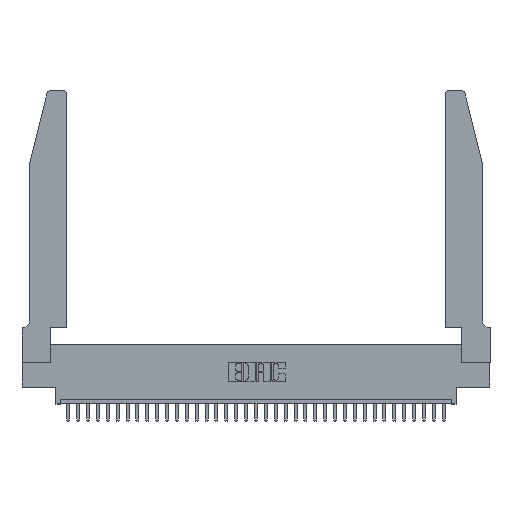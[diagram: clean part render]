
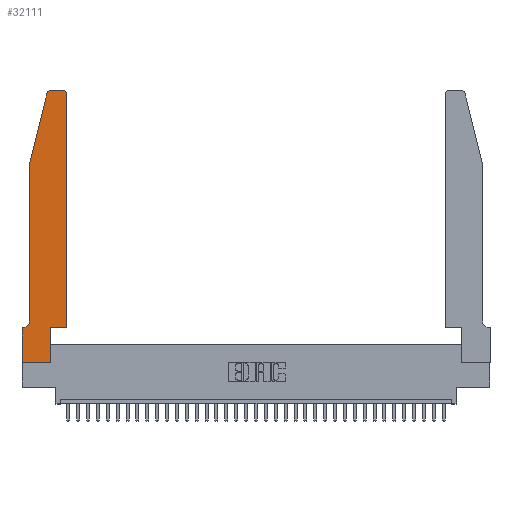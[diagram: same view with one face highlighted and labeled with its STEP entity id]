
A CAD part, top view. The second image highlights one B-rep face of the part: STEP entity #32111.
In plain terms, the highlighted planar face has unit normal (0, 0, 1).
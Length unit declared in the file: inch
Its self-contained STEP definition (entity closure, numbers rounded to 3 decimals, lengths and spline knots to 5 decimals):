
#231 = LINE ( 'NONE', #25158, #9953 ) ;
#695 = EDGE_CURVE ( 'NONE', #13591, #30207, #231, .T. ) ;
#723 = VERTEX_POINT ( 'NONE', #19340 ) ;
#740 = VERTEX_POINT ( 'NONE', #11806 ) ;
#1119 = EDGE_CURVE ( 'NONE', #15987, #22482, #8216, .T. ) ;
#1306 = VECTOR ( 'NONE', #20928, 39.37008 ) ;
#1535 = CARTESIAN_POINT ( 'NONE',  ( 0.0755, 2., 0.37 ) ) ;
#1785 = CARTESIAN_POINT ( 'NONE',  ( 0.4205, 2.72, 0.37 ) ) ;
#2062 = CARTESIAN_POINT ( 'NONE',  ( 0.2865, 0.35, 0.37 ) ) ;
#2480 = ORIENTED_EDGE ( 'NONE', *, *, #1119, .T. ) ;
#2664 = DIRECTION ( 'NONE',  ( 1., 0., 0. ) ) ;
#2764 = DIRECTION ( 'NONE',  ( 0., 0., 1. ) ) ;
#2852 = VERTEX_POINT ( 'NONE', #3169 ) ;
#2932 = EDGE_CURVE ( 'NONE', #723, #13591, #22415, .T. ) ;
#3169 = CARTESIAN_POINT ( 'NONE',  ( 0.0055, 0.35, 0.37 ) ) ;
#3414 = ORIENTED_EDGE ( 'NONE', *, *, #4445, .T. ) ;
#3510 = CARTESIAN_POINT ( 'NONE',  ( 0.25487, 2.72718, 0.37 ) ) ;
#3729 = AXIS2_PLACEMENT_3D ( 'NONE', #18151, #2764, #2664 ) ;
#4177 = EDGE_CURVE ( 'NONE', #9342, #21267, #10605, .T. ) ;
#4374 = DIRECTION ( 'NONE',  ( 0., -1., 0. ) ) ;
#4445 = EDGE_CURVE ( 'NONE', #21267, #28491, #19620, .T. ) ;
#4500 = DIRECTION ( 'NONE',  ( 0., 0., 1. ) ) ;
#4978 = CARTESIAN_POINT ( 'NONE',  ( 0.4505, 0.35, 0.37 ) ) ;
#4989 = ORIENTED_EDGE ( 'NONE', *, *, #17457, .T. ) ;
#5210 = DIRECTION ( 'NONE',  ( 1., 0., 0. ) ) ;
#6478 = CARTESIAN_POINT ( 'NONE',  ( 0.4205, 2.75, 0.37 ) ) ;
#7223 = CARTESIAN_POINT ( 'NONE',  ( 0.4505, 0.35, 0.37 ) ) ;
#7602 = AXIS2_PLACEMENT_3D ( 'NONE', #14707, #10553, #5210 ) ;
#8216 = LINE ( 'NONE', #7223, #17879 ) ;
#8486 = ORIENTED_EDGE ( 'NONE', *, *, #9682, .T. ) ;
#8666 = DIRECTION ( 'NONE',  ( 1., 0., 0. ) ) ;
#9342 = VERTEX_POINT ( 'NONE', #6478 ) ;
#9413 = VECTOR ( 'NONE', #20097, 39.37008 ) ;
#9682 = EDGE_CURVE ( 'NONE', #740, #2852, #26356, .T. ) ;
#9953 = VECTOR ( 'NONE', #8666, 39.37008 ) ;
#10314 = EDGE_LOOP ( 'NONE', ( #19942, #3414, #25070, #4989, #8486, #24636, #27515, #32850, #16488, #33091, #2480, #21799 ) ) ;
#10553 = DIRECTION ( 'NONE',  ( 0., 0., 1. ) ) ;
#10605 = LINE ( 'NONE', #12076, #16059 ) ;
#10651 = VECTOR ( 'NONE', #12559, 39.37008 ) ;
#11393 = CARTESIAN_POINT ( 'NONE',  ( 0., 0., 0.37 ) ) ;
#11806 = CARTESIAN_POINT ( 'NONE',  ( 0.0755, 0.42, 0.37 ) ) ;
#12007 = EDGE_CURVE ( 'NONE', #30207, #16808, #25762, .T. ) ;
#12076 = CARTESIAN_POINT ( 'NONE',  ( 0.2605, 2.75, 0.37 ) ) ;
#12324 = EDGE_CURVE ( 'NONE', #28491, #19335, #12341, .T. ) ;
#12341 = LINE ( 'NONE', #22961, #10651 ) ;
#12559 = DIRECTION ( 'NONE',  ( -0.239, -0.971, 0. ) ) ;
#12579 = DIRECTION ( 'NONE',  ( -1., 0., 0. ) ) ;
#13591 = VERTEX_POINT ( 'NONE', #11393 ) ;
#13728 = PLANE ( 'NONE',  #3729 ) ;
#14381 = CARTESIAN_POINT ( 'NONE',  ( 0., 0., 0.37 ) ) ;
#14707 = CARTESIAN_POINT ( 'NONE',  ( 0.284, 2.72, 0.37 ) ) ;
#14744 = CARTESIAN_POINT ( 'NONE',  ( 0.4505, 0.35, 0.37 ) ) ;
#14808 = VECTOR ( 'NONE', #23072, 39.37008 ) ;
#15380 = DIRECTION ( 'NONE',  ( 0., 1., 0. ) ) ;
#15719 = DIRECTION ( 'NONE',  ( 0., 1., 0. ) ) ;
#15987 = VERTEX_POINT ( 'NONE', #14744 ) ;
#16059 = VECTOR ( 'NONE', #20062, 39.37008 ) ;
#16488 = ORIENTED_EDGE ( 'NONE', *, *, #12007, .T. ) ;
#16808 = VERTEX_POINT ( 'NONE', #34144 ) ;
#16894 = LINE ( 'NONE', #33735, #14808 ) ;
#17280 = LINE ( 'NONE', #4978, #1306 ) ;
#17457 = EDGE_CURVE ( 'NONE', #19335, #740, #29896, .T. ) ;
#17879 = VECTOR ( 'NONE', #15719, 39.37008 ) ;
#18151 = CARTESIAN_POINT ( 'NONE',  ( 0., 0.35, 0.37 ) ) ;
#18416 = CARTESIAN_POINT ( 'NONE',  ( 0.4505, 2.72, 0.37 ) ) ;
#19335 = VERTEX_POINT ( 'NONE', #21433 ) ;
#19340 = CARTESIAN_POINT ( 'NONE',  ( 0., 0.35, 0.37 ) ) ;
#19620 = CIRCLE ( 'NONE', #7602, 0.03 ) ;
#19942 = ORIENTED_EDGE ( 'NONE', *, *, #4177, .T. ) ;
#20062 = DIRECTION ( 'NONE',  ( -1., 0., 0. ) ) ;
#20097 = DIRECTION ( 'NONE',  ( 0., -1., 0. ) ) ;
#20304 = DIRECTION ( 'NONE',  ( 0., 0., -1. ) ) ;
#20560 = CIRCLE ( 'NONE', #21873, 0.03 ) ;
#20928 = DIRECTION ( 'NONE',  ( 1., 0., 0. ) ) ;
#21165 = AXIS2_PLACEMENT_3D ( 'NONE', #22750, #20304, #12579 ) ;
#21267 = VERTEX_POINT ( 'NONE', #26312 ) ;
#21433 = CARTESIAN_POINT ( 'NONE',  ( 0.0755, 2., 0.37 ) ) ;
#21799 = ORIENTED_EDGE ( 'NONE', *, *, #28025, .T. ) ;
#21873 = AXIS2_PLACEMENT_3D ( 'NONE', #1785, #4500, #23376 ) ;
#22415 = LINE ( 'NONE', #14381, #9413 ) ;
#22482 = VERTEX_POINT ( 'NONE', #18416 ) ;
#22750 = CARTESIAN_POINT ( 'NONE',  ( 0.0055, 0.42, 0.37 ) ) ;
#22961 = CARTESIAN_POINT ( 'NONE',  ( 0.0755, 2., 0.37 ) ) ;
#23072 = DIRECTION ( 'NONE',  ( -1., 0., 0. ) ) ;
#23376 = DIRECTION ( 'NONE',  ( 1., 0., 0. ) ) ;
#24636 = ORIENTED_EDGE ( 'NONE', *, *, #25432, .T. ) ;
#25070 = ORIENTED_EDGE ( 'NONE', *, *, #12324, .T. ) ;
#25158 = CARTESIAN_POINT ( 'NONE',  ( 0., 0., 0.37 ) ) ;
#25432 = EDGE_CURVE ( 'NONE', #2852, #723, #16894, .T. ) ;
#25762 = LINE ( 'NONE', #2062, #32890 ) ;
#26312 = CARTESIAN_POINT ( 'NONE',  ( 0.284, 2.75, 0.37 ) ) ;
#26356 = CIRCLE ( 'NONE', #21165, 0.07 ) ;
#27381 = VECTOR ( 'NONE', #4374, 39.37008 ) ;
#27515 = ORIENTED_EDGE ( 'NONE', *, *, #2932, .T. ) ;
#28025 = EDGE_CURVE ( 'NONE', #22482, #9342, #20560, .T. ) ;
#28491 = VERTEX_POINT ( 'NONE', #3510 ) ;
#29896 = LINE ( 'NONE', #1535, #27381 ) ;
#30207 = VERTEX_POINT ( 'NONE', #34379 ) ;
#32111 = ADVANCED_FACE ( 'NONE', ( #33720 ), #13728, .T. ) ;
#32850 = ORIENTED_EDGE ( 'NONE', *, *, #695, .T. ) ;
#32890 = VECTOR ( 'NONE', #15380, 39.37008 ) ;
#33073 = EDGE_CURVE ( 'NONE', #16808, #15987, #17280, .T. ) ;
#33091 = ORIENTED_EDGE ( 'NONE', *, *, #33073, .T. ) ;
#33720 = FACE_OUTER_BOUND ( 'NONE', #10314, .T. ) ;
#33735 = CARTESIAN_POINT ( 'NONE',  ( 0.0755, 0.35, 0.37 ) ) ;
#34144 = CARTESIAN_POINT ( 'NONE',  ( 0.2865, 0.35, 0.37 ) ) ;
#34379 = CARTESIAN_POINT ( 'NONE',  ( 0.2865, 0., 0.37 ) ) ;
